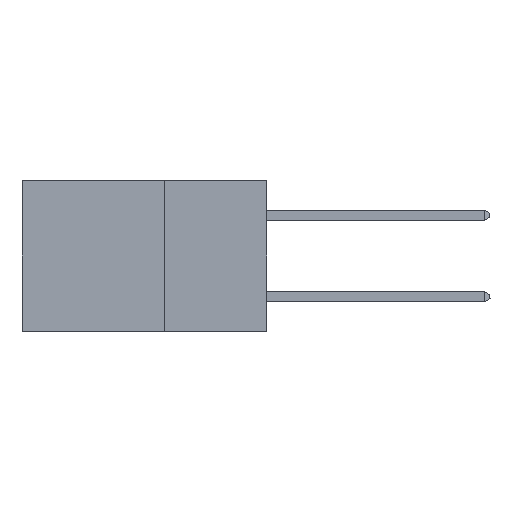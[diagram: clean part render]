
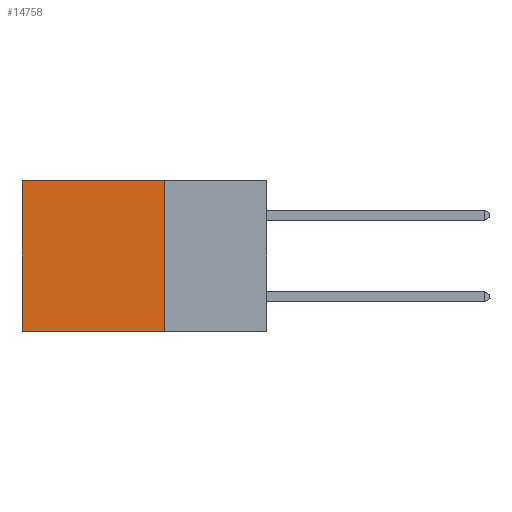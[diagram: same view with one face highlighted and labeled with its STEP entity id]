
A CAD part, left-side view. The second image highlights one B-rep face of the part: STEP entity #14758.
In plain terms, the highlighted planar face has unit normal (-1, 0, 0).
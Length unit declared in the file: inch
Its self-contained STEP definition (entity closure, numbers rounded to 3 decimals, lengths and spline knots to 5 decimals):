
#288 = CARTESIAN_POINT ( 'NONE',  ( 0.2875, 0.6, -0.37 ) ) ;
#2913 = DIRECTION ( 'NONE',  ( 0., 0., -1. ) ) ;
#3232 = DIRECTION ( 'NONE',  ( 0., 0., -1. ) ) ;
#3436 = CARTESIAN_POINT ( 'NONE',  ( 0.2875, 0.6, 0. ) ) ;
#4359 = VECTOR ( 'NONE', #25418, 39.37008 ) ;
#4469 = CARTESIAN_POINT ( 'NONE',  ( 0.2875, 0.25, -0.37 ) ) ;
#5376 = EDGE_CURVE ( 'NONE', #20974, #9166, #7983, .T. ) ;
#5663 = VECTOR ( 'NONE', #2913, 39.37008 ) ;
#6353 = LINE ( 'NONE', #11425, #11549 ) ;
#6737 = EDGE_LOOP ( 'NONE', ( #17046, #19191, #23944, #26988 ) ) ;
#7983 = LINE ( 'NONE', #4469, #4359 ) ;
#8409 = PLANE ( 'NONE',  #17810 ) ;
#9166 = VERTEX_POINT ( 'NONE', #288 ) ;
#9195 = DIRECTION ( 'NONE',  ( 0., 1., 0. ) ) ;
#9245 = CARTESIAN_POINT ( 'NONE',  ( 0.2875, 0.25, 0. ) ) ;
#11159 = EDGE_CURVE ( 'NONE', #22861, #9166, #18373, .T. ) ;
#11425 = CARTESIAN_POINT ( 'NONE',  ( 0.2875, 0.25, 0. ) ) ;
#11549 = VECTOR ( 'NONE', #3232, 39.37008 ) ;
#12252 = DIRECTION ( 'NONE',  ( 0., 0., -1. ) ) ;
#13209 = CARTESIAN_POINT ( 'NONE',  ( 0.2875, 0.6, 0. ) ) ;
#14758 = ADVANCED_FACE ( 'NONE', ( #22807 ), #8409, .F. ) ;
#15039 = LINE ( 'NONE', #21625, #22180 ) ;
#15094 = VERTEX_POINT ( 'NONE', #9245 ) ;
#17046 = ORIENTED_EDGE ( 'NONE', *, *, #11159, .T. ) ;
#17810 = AXIS2_PLACEMENT_3D ( 'NONE', #22773, #24690, #12252 ) ;
#18373 = LINE ( 'NONE', #3436, #5663 ) ;
#19191 = ORIENTED_EDGE ( 'NONE', *, *, #5376, .F. ) ;
#19977 = CARTESIAN_POINT ( 'NONE',  ( 0.2875, 0.25, -0.37 ) ) ;
#20974 = VERTEX_POINT ( 'NONE', #19977 ) ;
#21625 = CARTESIAN_POINT ( 'NONE',  ( 0.2875, 0.25, 0. ) ) ;
#22180 = VECTOR ( 'NONE', #9195, 39.37008 ) ;
#22773 = CARTESIAN_POINT ( 'NONE',  ( 0.2875, 0.25, 0. ) ) ;
#22807 = FACE_OUTER_BOUND ( 'NONE', #6737, .T. ) ;
#22861 = VERTEX_POINT ( 'NONE', #13209 ) ;
#22939 = EDGE_CURVE ( 'NONE', #15094, #22861, #15039, .T. ) ;
#23944 = ORIENTED_EDGE ( 'NONE', *, *, #24365, .F. ) ;
#24365 = EDGE_CURVE ( 'NONE', #15094, #20974, #6353, .T. ) ;
#24690 = DIRECTION ( 'NONE',  ( 1., 0., 0. ) ) ;
#25418 = DIRECTION ( 'NONE',  ( 0., 1., 0. ) ) ;
#26988 = ORIENTED_EDGE ( 'NONE', *, *, #22939, .T. ) ;
